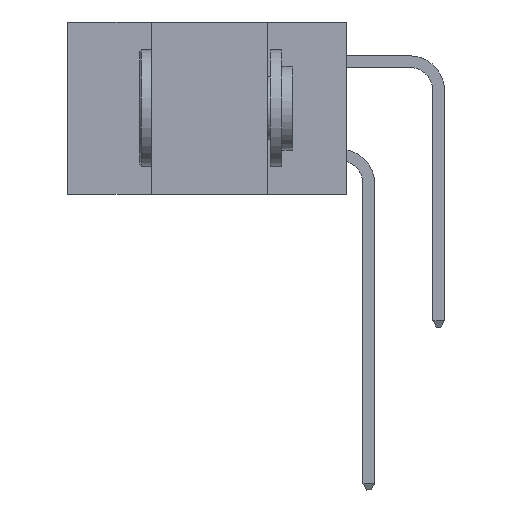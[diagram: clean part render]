
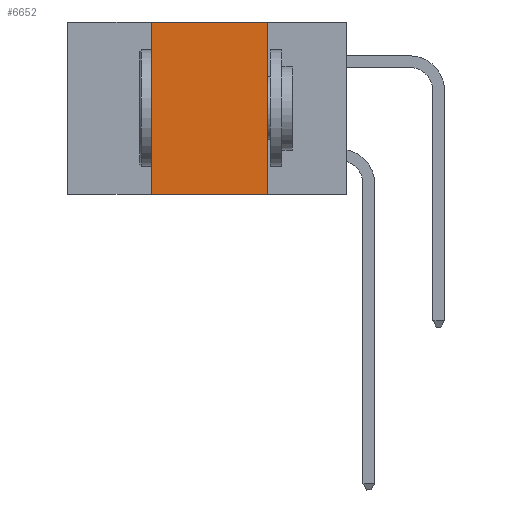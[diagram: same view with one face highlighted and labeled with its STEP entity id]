
A CAD part, left-side view. The second image highlights one B-rep face of the part: STEP entity #6652.
In plain terms, the highlighted planar face has unit normal (-1, 0, 0).
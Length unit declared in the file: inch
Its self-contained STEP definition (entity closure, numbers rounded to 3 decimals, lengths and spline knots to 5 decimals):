
#36 = DIRECTION ( 'NONE',  ( 1., 0., 0. ) ) ;
#475 = LINE ( 'NONE', #11704, #14464 ) ;
#1338 = EDGE_CURVE ( 'NONE', #7918, #8114, #16991, .T. ) ;
#3037 = LINE ( 'NONE', #5224, #17669 ) ;
#3273 = ORIENTED_EDGE ( 'NONE', *, *, #12329, .F. ) ;
#3309 = ORIENTED_EDGE ( 'NONE', *, *, #11693, .F. ) ;
#3449 = ORIENTED_EDGE ( 'NONE', *, *, #1338, .F. ) ;
#3594 = ORIENTED_EDGE ( 'NONE', *, *, #10745, .T. ) ;
#4009 = FACE_OUTER_BOUND ( 'NONE', #10595, .T. ) ;
#4584 = CARTESIAN_POINT ( 'NONE',  ( 0., 0.6, 0. ) ) ;
#5224 = CARTESIAN_POINT ( 'NONE',  ( 0., 0.6, 0. ) ) ;
#6034 = PLANE ( 'NONE',  #9293 ) ;
#6241 = VERTEX_POINT ( 'NONE', #10569 ) ;
#6652 = ADVANCED_FACE ( 'NONE', ( #4009 ), #6034, .F. ) ;
#6660 = DIRECTION ( 'NONE',  ( 0., -1., 0. ) ) ;
#6696 = DIRECTION ( 'NONE',  ( 0., 0., -1. ) ) ;
#6752 = CARTESIAN_POINT ( 'NONE',  ( 0., 0.17, -0.37 ) ) ;
#7918 = VERTEX_POINT ( 'NONE', #13342 ) ;
#8114 = VERTEX_POINT ( 'NONE', #9503 ) ;
#8850 = VERTEX_POINT ( 'NONE', #6752 ) ;
#9293 = AXIS2_PLACEMENT_3D ( 'NONE', #4584, #36, #15938 ) ;
#9503 = CARTESIAN_POINT ( 'NONE',  ( 0., 0.42, 0. ) ) ;
#10569 = CARTESIAN_POINT ( 'NONE',  ( 0., 0.17, 0. ) ) ;
#10595 = EDGE_LOOP ( 'NONE', ( #3273, #3309, #3449, #3594 ) ) ;
#10745 = EDGE_CURVE ( 'NONE', #7918, #8850, #475, .T. ) ;
#10859 = VECTOR ( 'NONE', #6696, 39.37008 ) ;
#11693 = EDGE_CURVE ( 'NONE', #8114, #6241, #3037, .T. ) ;
#11704 = CARTESIAN_POINT ( 'NONE',  ( 0., 0.6, -0.37 ) ) ;
#12329 = EDGE_CURVE ( 'NONE', #6241, #8850, #18283, .T. ) ;
#12831 = VECTOR ( 'NONE', #17283, 39.37008 ) ;
#13126 = DIRECTION ( 'NONE',  ( 0., -1., 0. ) ) ;
#13342 = CARTESIAN_POINT ( 'NONE',  ( 0., 0.42, -0.37 ) ) ;
#14464 = VECTOR ( 'NONE', #13126, 39.37008 ) ;
#15938 = DIRECTION ( 'NONE',  ( 0., 0., -1. ) ) ;
#16574 = CARTESIAN_POINT ( 'NONE',  ( 0., 0.17, 0. ) ) ;
#16991 = LINE ( 'NONE', #17201, #12831 ) ;
#17201 = CARTESIAN_POINT ( 'NONE',  ( 0., 0.42, 0. ) ) ;
#17283 = DIRECTION ( 'NONE',  ( 0., 0., 1. ) ) ;
#17669 = VECTOR ( 'NONE', #6660, 39.37008 ) ;
#18283 = LINE ( 'NONE', #16574, #10859 ) ;
